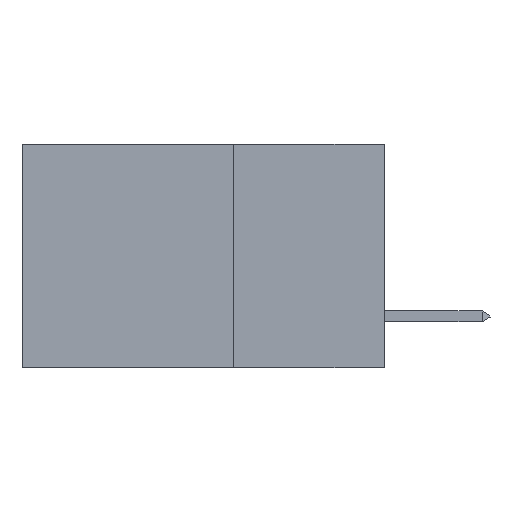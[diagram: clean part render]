
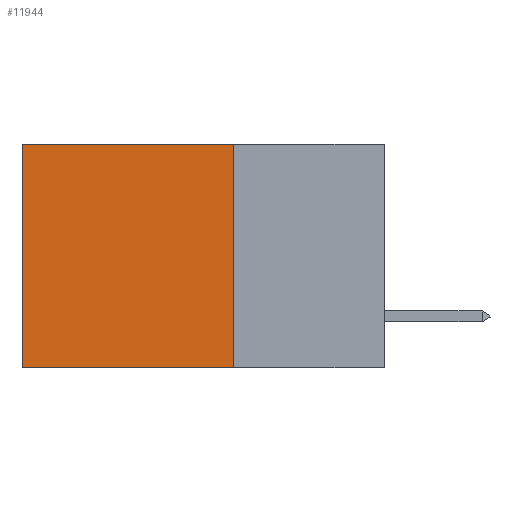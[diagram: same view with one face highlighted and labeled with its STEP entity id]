
A CAD part, left-side view. The second image highlights one B-rep face of the part: STEP entity #11944.
In plain terms, the highlighted planar face has unit normal (-1, 0, 0).
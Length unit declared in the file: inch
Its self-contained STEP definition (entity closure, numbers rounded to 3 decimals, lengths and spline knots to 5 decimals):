
#168 = CARTESIAN_POINT ( 'NONE',  ( 0.2875, 0.25, 0. ) ) ;
#1240 = FACE_OUTER_BOUND ( 'NONE', #2652, .T. ) ;
#2341 = DIRECTION ( 'NONE',  ( 1., 0., 0. ) ) ;
#2652 = EDGE_LOOP ( 'NONE', ( #4212, #2742, #14915, #12816 ) ) ;
#2674 = LINE ( 'NONE', #9929, #9958 ) ;
#2742 = ORIENTED_EDGE ( 'NONE', *, *, #4004, .F. ) ;
#2952 = VECTOR ( 'NONE', #7339, 39.37008 ) ;
#2978 = DIRECTION ( 'NONE',  ( 0., 0., -1. ) ) ;
#3109 = VECTOR ( 'NONE', #14046, 39.37008 ) ;
#4004 = EDGE_CURVE ( 'NONE', #5468, #4115, #6577, .T. ) ;
#4115 = VERTEX_POINT ( 'NONE', #8784 ) ;
#4212 = ORIENTED_EDGE ( 'NONE', *, *, #7063, .T. ) ;
#4497 = EDGE_CURVE ( 'NONE', #10241, #12258, #10032, .T. ) ;
#5468 = VERTEX_POINT ( 'NONE', #6155 ) ;
#6155 = CARTESIAN_POINT ( 'NONE',  ( 0.2875, 0.25, -0.37 ) ) ;
#6577 = LINE ( 'NONE', #9794, #2952 ) ;
#7063 = EDGE_CURVE ( 'NONE', #12258, #4115, #14967, .T. ) ;
#7339 = DIRECTION ( 'NONE',  ( 0., 1., 0. ) ) ;
#8729 = DIRECTION ( 'NONE',  ( 0., 0., -1. ) ) ;
#8784 = CARTESIAN_POINT ( 'NONE',  ( 0.2875, 0.6, -0.37 ) ) ;
#9794 = CARTESIAN_POINT ( 'NONE',  ( 0.2875, 0.25, -0.37 ) ) ;
#9929 = CARTESIAN_POINT ( 'NONE',  ( 0.2875, 0.25, 0. ) ) ;
#9948 = CARTESIAN_POINT ( 'NONE',  ( 0.2875, 0.6, 0. ) ) ;
#9958 = VECTOR ( 'NONE', #8729, 39.37008 ) ;
#10032 = LINE ( 'NONE', #12874, #3109 ) ;
#10241 = VERTEX_POINT ( 'NONE', #11972 ) ;
#10506 = EDGE_CURVE ( 'NONE', #10241, #5468, #2674, .T. ) ;
#11296 = AXIS2_PLACEMENT_3D ( 'NONE', #168, #2341, #11708 ) ;
#11708 = DIRECTION ( 'NONE',  ( 0., 0., -1. ) ) ;
#11944 = ADVANCED_FACE ( 'NONE', ( #1240 ), #13934, .F. ) ;
#11972 = CARTESIAN_POINT ( 'NONE',  ( 0.2875, 0.25, 0. ) ) ;
#12258 = VERTEX_POINT ( 'NONE', #12896 ) ;
#12816 = ORIENTED_EDGE ( 'NONE', *, *, #4497, .T. ) ;
#12874 = CARTESIAN_POINT ( 'NONE',  ( 0.2875, 0.25, 0. ) ) ;
#12896 = CARTESIAN_POINT ( 'NONE',  ( 0.2875, 0.6, 0. ) ) ;
#13934 = PLANE ( 'NONE',  #11296 ) ;
#14046 = DIRECTION ( 'NONE',  ( 0., 1., 0. ) ) ;
#14419 = VECTOR ( 'NONE', #2978, 39.37008 ) ;
#14915 = ORIENTED_EDGE ( 'NONE', *, *, #10506, .F. ) ;
#14967 = LINE ( 'NONE', #9948, #14419 ) ;
